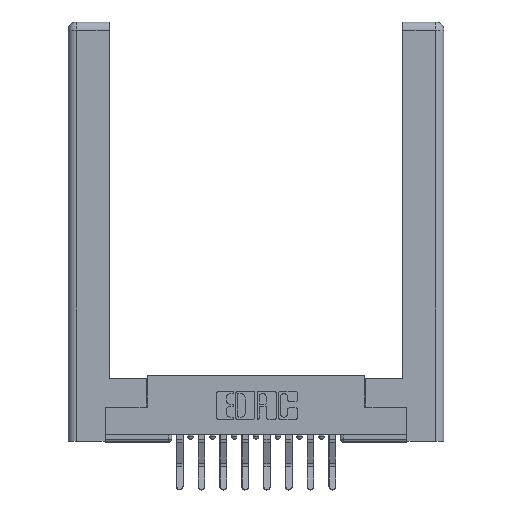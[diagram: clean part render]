
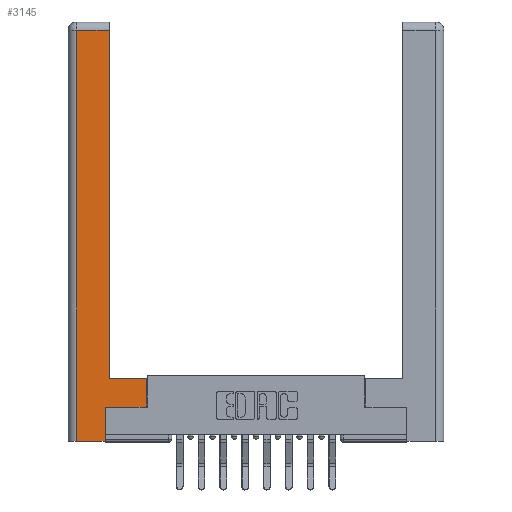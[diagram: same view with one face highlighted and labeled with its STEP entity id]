
A CAD part, top view. The second image highlights one B-rep face of the part: STEP entity #3145.
In plain terms, the highlighted planar face has unit normal (0, 0, 1).
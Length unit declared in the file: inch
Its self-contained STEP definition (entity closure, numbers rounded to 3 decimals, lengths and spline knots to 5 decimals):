
#543 = DIRECTION ( 'NONE',  ( -1., 0., 0. ) ) ;
#724 = VERTEX_POINT ( 'NONE', #12786 ) ;
#737 = CARTESIAN_POINT ( 'NONE',  ( 0.565, 0.45, 0. ) ) ;
#767 = LINE ( 'NONE', #13834, #9919 ) ;
#1114 = EDGE_CURVE ( 'NONE', #11188, #11573, #767, .T. ) ;
#1115 = ORIENTED_EDGE ( 'NONE', *, *, #12265, .T. ) ;
#1255 = LINE ( 'NONE', #1555, #12103 ) ;
#1318 = VECTOR ( 'NONE', #6409, 39.37008 ) ;
#1555 = CARTESIAN_POINT ( 'NONE',  ( 0.0615, 2.94, 0. ) ) ;
#1633 = EDGE_CURVE ( 'NONE', #3178, #11188, #6016, .T. ) ;
#1667 = CARTESIAN_POINT ( 'NONE',  ( 0.565, 0.245, 0. ) ) ;
#1744 = FACE_OUTER_BOUND ( 'NONE', #9173, .T. ) ;
#2281 = VECTOR ( 'NONE', #13521, 39.37008 ) ;
#3021 = DIRECTION ( 'NONE',  ( 0., -1., 0. ) ) ;
#3088 = CARTESIAN_POINT ( 'NONE',  ( 0., 0., 0. ) ) ;
#3145 = ADVANCED_FACE ( 'NONE', ( #1744 ), #11710, .F. ) ;
#3178 = VERTEX_POINT ( 'NONE', #14060 ) ;
#3856 = ORIENTED_EDGE ( 'NONE', *, *, #13760, .T. ) ;
#4075 = EDGE_CURVE ( 'NONE', #11573, #9945, #6953, .T. ) ;
#4173 = CARTESIAN_POINT ( 'NONE',  ( 0.0615, 0., 0. ) ) ;
#4222 = CARTESIAN_POINT ( 'NONE',  ( 0.295, 3., 0. ) ) ;
#4402 = EDGE_CURVE ( 'NONE', #9928, #724, #1255, .T. ) ;
#5408 = ORIENTED_EDGE ( 'NONE', *, *, #1633, .T. ) ;
#5425 = ORIENTED_EDGE ( 'NONE', *, *, #4402, .T. ) ;
#5739 = ORIENTED_EDGE ( 'NONE', *, *, #9086, .T. ) ;
#5821 = ORIENTED_EDGE ( 'NONE', *, *, #1114, .T. ) ;
#5834 = ORIENTED_EDGE ( 'NONE', *, *, #9851, .T. ) ;
#6016 = LINE ( 'NONE', #1667, #2281 ) ;
#6085 = CARTESIAN_POINT ( 'NONE',  ( 0.295, 0.45, 0. ) ) ;
#6271 = DIRECTION ( 'NONE',  ( -1., 0., 0. ) ) ;
#6409 = DIRECTION ( 'NONE',  ( 0., 1., 0. ) ) ;
#6462 = DIRECTION ( 'NONE',  ( 0., 1., 0. ) ) ;
#6609 = VECTOR ( 'NONE', #11163, 39.37008 ) ;
#6654 = CARTESIAN_POINT ( 'NONE',  ( 0.0615, 0., 0. ) ) ;
#6831 = CARTESIAN_POINT ( 'NONE',  ( 0.265, 0., 0. ) ) ;
#6953 = LINE ( 'NONE', #11118, #6609 ) ;
#7083 = CARTESIAN_POINT ( 'NONE',  ( 0.265, 0.245, 0. ) ) ;
#7137 = CARTESIAN_POINT ( 'NONE',  ( 0.295, 2.94, 0. ) ) ;
#8045 = VECTOR ( 'NONE', #11437, 39.37008 ) ;
#8340 = VERTEX_POINT ( 'NONE', #6654 ) ;
#9086 = EDGE_CURVE ( 'NONE', #8340, #12165, #9255, .T. ) ;
#9173 = EDGE_LOOP ( 'NONE', ( #3856, #5425, #1115, #5739, #5834, #5408, #5821, #10847 ) ) ;
#9255 = LINE ( 'NONE', #6831, #12311 ) ;
#9323 = LINE ( 'NONE', #4173, #11860 ) ;
#9684 = DIRECTION ( 'NONE',  ( 0., 0., -1. ) ) ;
#9851 = EDGE_CURVE ( 'NONE', #12165, #3178, #13844, .T. ) ;
#9919 = VECTOR ( 'NONE', #6462, 39.37008 ) ;
#9928 = VERTEX_POINT ( 'NONE', #7137 ) ;
#9945 = VERTEX_POINT ( 'NONE', #6085 ) ;
#10847 = ORIENTED_EDGE ( 'NONE', *, *, #4075, .T. ) ;
#10918 = CARTESIAN_POINT ( 'NONE',  ( 0.565, 0.245, 0. ) ) ;
#11080 = DIRECTION ( 'NONE',  ( 1., 0., 0. ) ) ;
#11118 = CARTESIAN_POINT ( 'NONE',  ( 0.295, 0.45, 0. ) ) ;
#11163 = DIRECTION ( 'NONE',  ( -1., 0., 0. ) ) ;
#11188 = VERTEX_POINT ( 'NONE', #10918 ) ;
#11313 = LINE ( 'NONE', #4222, #1318 ) ;
#11437 = DIRECTION ( 'NONE',  ( 0., 1., 0. ) ) ;
#11573 = VERTEX_POINT ( 'NONE', #737 ) ;
#11710 = PLANE ( 'NONE',  #13887 ) ;
#11860 = VECTOR ( 'NONE', #3021, 39.37008 ) ;
#12103 = VECTOR ( 'NONE', #543, 39.37008 ) ;
#12165 = VERTEX_POINT ( 'NONE', #13726 ) ;
#12265 = EDGE_CURVE ( 'NONE', #724, #8340, #9323, .T. ) ;
#12311 = VECTOR ( 'NONE', #11080, 39.37008 ) ;
#12786 = CARTESIAN_POINT ( 'NONE',  ( 0.0615, 2.94, 0. ) ) ;
#13521 = DIRECTION ( 'NONE',  ( 1., 0., 0. ) ) ;
#13726 = CARTESIAN_POINT ( 'NONE',  ( 0.265, 0., 0. ) ) ;
#13760 = EDGE_CURVE ( 'NONE', #9945, #9928, #11313, .T. ) ;
#13834 = CARTESIAN_POINT ( 'NONE',  ( 0.565, 0.45, 0. ) ) ;
#13844 = LINE ( 'NONE', #7083, #8045 ) ;
#13887 = AXIS2_PLACEMENT_3D ( 'NONE', #3088, #9684, #6271 ) ;
#14060 = CARTESIAN_POINT ( 'NONE',  ( 0.265, 0.245, 0. ) ) ;
